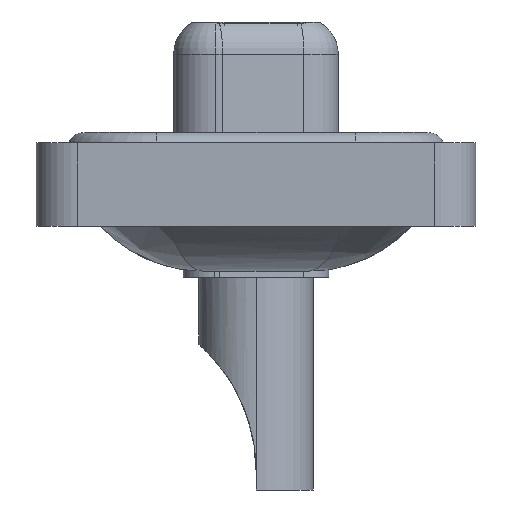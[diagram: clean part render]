
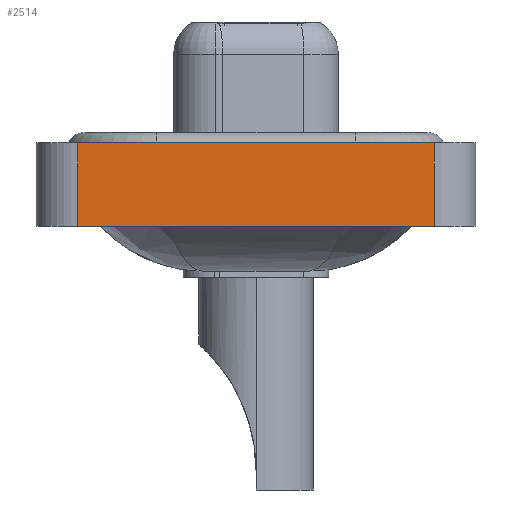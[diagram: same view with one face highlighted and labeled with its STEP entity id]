
A CAD part, left-side view. The second image highlights one B-rep face of the part: STEP entity #2514.
In plain terms, the highlighted planar face has unit normal (-1, 0, 0).
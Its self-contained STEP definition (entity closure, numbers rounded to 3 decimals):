
#1003 = VERTEX_POINT ( 'NONE', #4444 ) ;
#1041 = EDGE_CURVE ( 'NONE', #12496, #1003, #7415, .T. ) ;
#2108 = PLANE ( 'NONE',  #14807 ) ;
#2514 = ADVANCED_FACE ( 'NONE', ( #3666 ), #2108, .T. ) ;
#3440 = CARTESIAN_POINT ( 'NONE',  ( -7.25, -8.55, -3.6 ) ) ;
#3666 = FACE_OUTER_BOUND ( 'NONE', #4067, .T. ) ;
#4015 = ORIENTED_EDGE ( 'NONE', *, *, #5052, .F. ) ;
#4067 = EDGE_LOOP ( 'NONE', ( #8321, #4015, #11311, #6403 ) ) ;
#4444 = CARTESIAN_POINT ( 'NONE',  ( -7.25, -8.55, -3.6 ) ) ;
#4831 = CARTESIAN_POINT ( 'NONE',  ( -7.25, 8.55, -3.6 ) ) ;
#5052 = EDGE_CURVE ( 'NONE', #16497, #15620, #16483, .T. ) ;
#6403 = ORIENTED_EDGE ( 'NONE', *, *, #1041, .T. ) ;
#6408 = EDGE_CURVE ( 'NONE', #12496, #16497, #15121, .T. ) ;
#6413 = DIRECTION ( 'NONE',  ( 0., -1., 0. ) ) ;
#7248 = CARTESIAN_POINT ( 'NONE',  ( -7.25, 8.55, -3.6 ) ) ;
#7326 = CARTESIAN_POINT ( 'NONE',  ( -7.25, -8.55, -3.6 ) ) ;
#7415 = LINE ( 'NONE', #7326, #15042 ) ;
#8310 = VECTOR ( 'NONE', #13811, 1000. ) ;
#8321 = ORIENTED_EDGE ( 'NONE', *, *, #10229, .T. ) ;
#8812 = CARTESIAN_POINT ( 'NONE',  ( -7.25, 8.55, 0.4 ) ) ;
#8858 = CARTESIAN_POINT ( 'NONE',  ( -7.25, -8.55, -3.6 ) ) ;
#10229 = EDGE_CURVE ( 'NONE', #1003, #15620, #11289, .T. ) ;
#10437 = VECTOR ( 'NONE', #6413, 1000. ) ;
#11289 = LINE ( 'NONE', #3440, #14167 ) ;
#11311 = ORIENTED_EDGE ( 'NONE', *, *, #6408, .F. ) ;
#12462 = DIRECTION ( 'NONE',  ( -1., 0., 0. ) ) ;
#12496 = VERTEX_POINT ( 'NONE', #7248 ) ;
#13472 = CARTESIAN_POINT ( 'NONE',  ( -7.25, -8.55, 0.4 ) ) ;
#13728 = CARTESIAN_POINT ( 'NONE',  ( -7.25, -8.55, 0.4 ) ) ;
#13765 = DIRECTION ( 'NONE',  ( 0., 0., 1. ) ) ;
#13811 = DIRECTION ( 'NONE',  ( 0., 0., 1. ) ) ;
#14167 = VECTOR ( 'NONE', #14206, 1000. ) ;
#14206 = DIRECTION ( 'NONE',  ( 0., 0., 1. ) ) ;
#14807 = AXIS2_PLACEMENT_3D ( 'NONE', #8858, #12462, #13765 ) ;
#15042 = VECTOR ( 'NONE', #16600, 1000. ) ;
#15121 = LINE ( 'NONE', #4831, #8310 ) ;
#15620 = VERTEX_POINT ( 'NONE', #13472 ) ;
#16483 = LINE ( 'NONE', #13728, #10437 ) ;
#16497 = VERTEX_POINT ( 'NONE', #8812 ) ;
#16600 = DIRECTION ( 'NONE',  ( 0., -1., 0. ) ) ;
